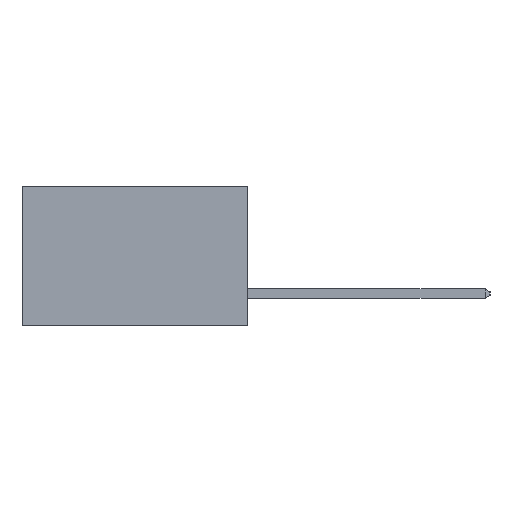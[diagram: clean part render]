
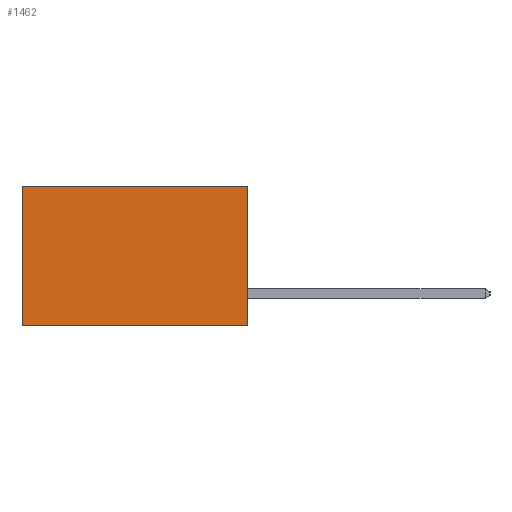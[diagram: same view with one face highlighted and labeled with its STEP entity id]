
A CAD part, left-side view. The second image highlights one B-rep face of the part: STEP entity #1462.
In plain terms, the highlighted planar face has unit normal (-1, 0, 0).
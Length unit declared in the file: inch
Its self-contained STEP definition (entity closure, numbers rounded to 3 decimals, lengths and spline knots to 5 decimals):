
#703 = ORIENTED_EDGE ( 'NONE', *, *, #8702, .T. ) ;
#942 = CARTESIAN_POINT ( 'NONE',  ( 0.2615, 0.6, -0.37 ) ) ;
#1057 = DIRECTION ( 'NONE',  ( 0., 0., -1. ) ) ;
#1366 = DIRECTION ( 'NONE',  ( 0., 0., -1. ) ) ;
#1462 = ADVANCED_FACE ( 'NONE', ( #5918 ), #17961, .F. ) ;
#2235 = LINE ( 'NONE', #16190, #9520 ) ;
#2240 = CARTESIAN_POINT ( 'NONE',  ( 0.2615, 0.6, -0.37 ) ) ;
#2586 = CARTESIAN_POINT ( 'NONE',  ( 0.2615, 0., -0.37 ) ) ;
#2630 = CARTESIAN_POINT ( 'NONE',  ( 0.2615, 0., -0.37 ) ) ;
#2772 = AXIS2_PLACEMENT_3D ( 'NONE', #2630, #13173, #19896 ) ;
#3886 = VERTEX_POINT ( 'NONE', #12750 ) ;
#4010 = VECTOR ( 'NONE', #1057, 39.37008 ) ;
#5084 = LINE ( 'NONE', #7792, #13227 ) ;
#5338 = ORIENTED_EDGE ( 'NONE', *, *, #8218, .F. ) ;
#5759 = VECTOR ( 'NONE', #1366, 39.37008 ) ;
#5918 = FACE_OUTER_BOUND ( 'NONE', #10344, .T. ) ;
#7792 = CARTESIAN_POINT ( 'NONE',  ( 0.2615, 0., -0.37 ) ) ;
#7905 = DIRECTION ( 'NONE',  ( 0., 1., 0. ) ) ;
#8218 = EDGE_CURVE ( 'NONE', #3886, #14919, #5084, .T. ) ;
#8702 = EDGE_CURVE ( 'NONE', #12185, #14919, #13209, .T. ) ;
#9520 = VECTOR ( 'NONE', #16676, 39.37008 ) ;
#10344 = EDGE_LOOP ( 'NONE', ( #703, #5338, #18990, #20202 ) ) ;
#10552 = CARTESIAN_POINT ( 'NONE',  ( 0.2615, 0.6, 0. ) ) ;
#12185 = VERTEX_POINT ( 'NONE', #10552 ) ;
#12750 = CARTESIAN_POINT ( 'NONE',  ( 0.2615, 0., -0.37 ) ) ;
#13173 = DIRECTION ( 'NONE',  ( 1., 0., 0. ) ) ;
#13209 = LINE ( 'NONE', #942, #4010 ) ;
#13227 = VECTOR ( 'NONE', #7905, 39.37008 ) ;
#14272 = EDGE_CURVE ( 'NONE', #20477, #12185, #2235, .T. ) ;
#14878 = LINE ( 'NONE', #2586, #5759 ) ;
#14919 = VERTEX_POINT ( 'NONE', #2240 ) ;
#16190 = CARTESIAN_POINT ( 'NONE',  ( 0.2615, 0., 0. ) ) ;
#16676 = DIRECTION ( 'NONE',  ( 0., 1., 0. ) ) ;
#17121 = EDGE_CURVE ( 'NONE', #20477, #3886, #14878, .T. ) ;
#17961 = PLANE ( 'NONE',  #2772 ) ;
#18990 = ORIENTED_EDGE ( 'NONE', *, *, #17121, .F. ) ;
#19313 = CARTESIAN_POINT ( 'NONE',  ( 0.2615, 0., 0. ) ) ;
#19896 = DIRECTION ( 'NONE',  ( 0., 0., -1. ) ) ;
#20202 = ORIENTED_EDGE ( 'NONE', *, *, #14272, .T. ) ;
#20477 = VERTEX_POINT ( 'NONE', #19313 ) ;
